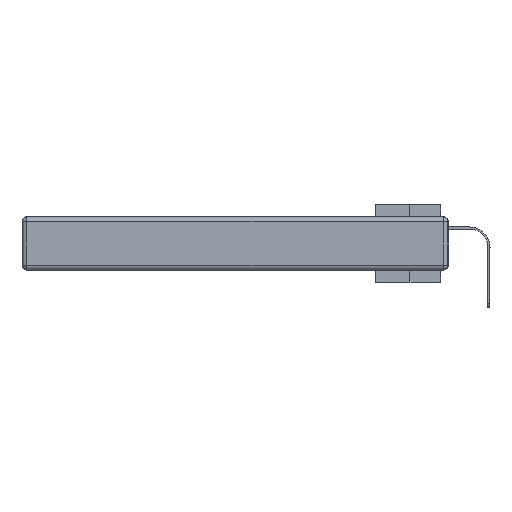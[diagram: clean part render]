
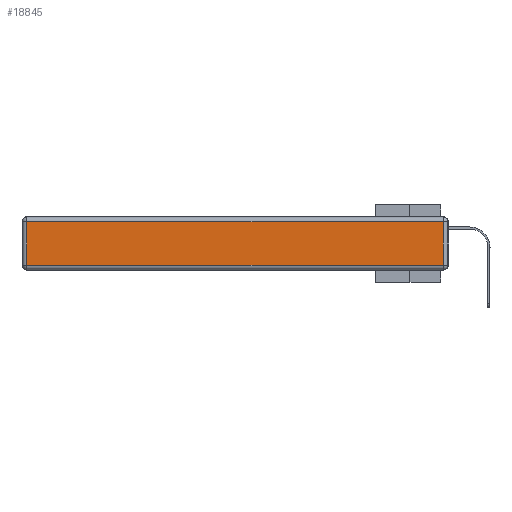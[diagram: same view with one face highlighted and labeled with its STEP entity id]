
A CAD part, left-side view. The second image highlights one B-rep face of the part: STEP entity #18845.
In plain terms, the highlighted planar face has unit normal (-1, 0, 0).
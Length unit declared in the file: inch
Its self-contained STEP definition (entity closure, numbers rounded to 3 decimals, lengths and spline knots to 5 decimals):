
#808 = VECTOR ( 'NONE', #2778, 39.37008 ) ;
#815 = DIRECTION ( 'NONE',  ( 0., 0., 1. ) ) ;
#1714 = VERTEX_POINT ( 'NONE', #21319 ) ;
#2778 = DIRECTION ( 'NONE',  ( 0., -1., 0. ) ) ;
#2843 = EDGE_CURVE ( 'NONE', #26711, #19533, #5591, .T. ) ;
#3238 = CARTESIAN_POINT ( 'NONE',  ( 0., 0., -0.313 ) ) ;
#3768 = FACE_OUTER_BOUND ( 'NONE', #9015, .T. ) ;
#4958 = EDGE_CURVE ( 'NONE', #19533, #18176, #7395, .T. ) ;
#5591 = LINE ( 'NONE', #3238, #808 ) ;
#5769 = CARTESIAN_POINT ( 'NONE',  ( 0., 2.72, -0.313 ) ) ;
#7395 = LINE ( 'NONE', #23942, #29494 ) ;
#8607 = DIRECTION ( 'NONE',  ( -1., 0., 0. ) ) ;
#9015 = EDGE_LOOP ( 'NONE', ( #10959, #25153, #27000, #18739 ) ) ;
#10046 = EDGE_CURVE ( 'NONE', #18176, #1714, #25633, .T. ) ;
#10959 = ORIENTED_EDGE ( 'NONE', *, *, #2843, .T. ) ;
#12315 = EDGE_CURVE ( 'NONE', #1714, #26711, #28973, .T. ) ;
#13284 = PLANE ( 'NONE',  #22847 ) ;
#15091 = CARTESIAN_POINT ( 'NONE',  ( 0., 2.72, -0.343 ) ) ;
#15990 = VECTOR ( 'NONE', #21793, 39.37008 ) ;
#17379 = CARTESIAN_POINT ( 'NONE',  ( 0., 0.03, -0.03 ) ) ;
#18176 = VERTEX_POINT ( 'NONE', #17379 ) ;
#18739 = ORIENTED_EDGE ( 'NONE', *, *, #12315, .T. ) ;
#18845 = ADVANCED_FACE ( 'NONE', ( #3768 ), #13284, .T. ) ;
#19533 = VERTEX_POINT ( 'NONE', #24241 ) ;
#19766 = CARTESIAN_POINT ( 'NONE',  ( 0., 2.75, -0.03 ) ) ;
#21319 = CARTESIAN_POINT ( 'NONE',  ( 0., 2.72, -0.03 ) ) ;
#21793 = DIRECTION ( 'NONE',  ( 0., 0., -1. ) ) ;
#22794 = CARTESIAN_POINT ( 'NONE',  ( 0., 0., -0.343 ) ) ;
#22847 = AXIS2_PLACEMENT_3D ( 'NONE', #22794, #8607, #815 ) ;
#22849 = VECTOR ( 'NONE', #29256, 39.37008 ) ;
#23942 = CARTESIAN_POINT ( 'NONE',  ( 0., 0.03, -0.343 ) ) ;
#24241 = CARTESIAN_POINT ( 'NONE',  ( 0., 0.03, -0.313 ) ) ;
#25153 = ORIENTED_EDGE ( 'NONE', *, *, #4958, .T. ) ;
#25633 = LINE ( 'NONE', #19766, #22849 ) ;
#26711 = VERTEX_POINT ( 'NONE', #5769 ) ;
#26731 = DIRECTION ( 'NONE',  ( 0., 0., 1. ) ) ;
#27000 = ORIENTED_EDGE ( 'NONE', *, *, #10046, .T. ) ;
#28973 = LINE ( 'NONE', #15091, #15990 ) ;
#29256 = DIRECTION ( 'NONE',  ( 0., 1., 0. ) ) ;
#29494 = VECTOR ( 'NONE', #26731, 39.37008 ) ;
